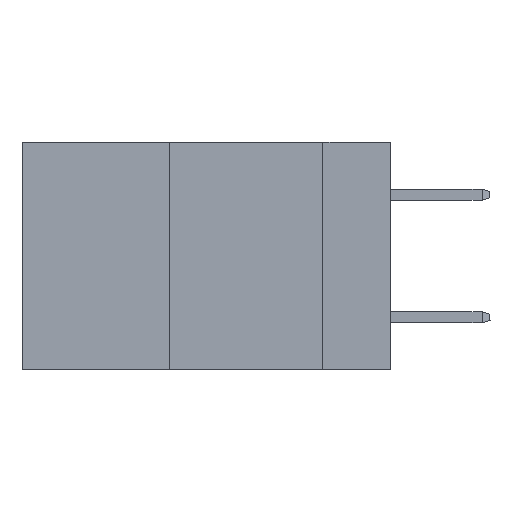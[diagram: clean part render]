
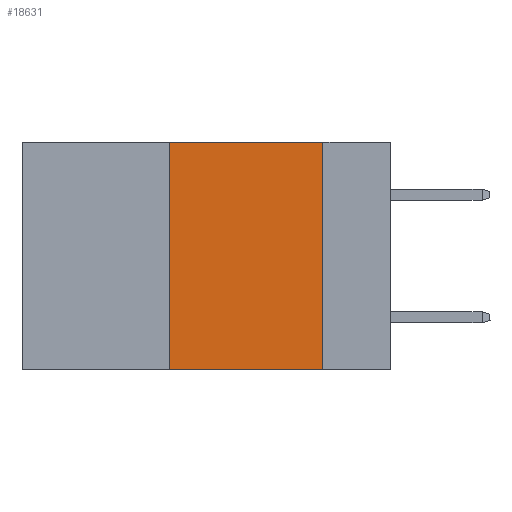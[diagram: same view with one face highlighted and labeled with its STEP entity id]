
A CAD part, left-side view. The second image highlights one B-rep face of the part: STEP entity #18631.
In plain terms, the highlighted planar face has unit normal (-1, 0, 0).
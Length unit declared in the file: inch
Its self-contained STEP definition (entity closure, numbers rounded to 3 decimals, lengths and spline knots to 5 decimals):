
#209 = CARTESIAN_POINT ( 'NONE',  ( 0., 0.6, -0.37 ) ) ;
#716 = EDGE_CURVE ( 'NONE', #15757, #21179, #43046, .T. ) ;
#982 = CARTESIAN_POINT ( 'NONE',  ( 0., 0.11, 0. ) ) ;
#2478 = LINE ( 'NONE', #23327, #38854 ) ;
#2744 = EDGE_LOOP ( 'NONE', ( #33488, #43455, #37711, #19907 ) ) ;
#6216 = CARTESIAN_POINT ( 'NONE',  ( 0., 0.36, -0.37 ) ) ;
#6504 = VERTEX_POINT ( 'NONE', #6216 ) ;
#7935 = VECTOR ( 'NONE', #11816, 39.37008 ) ;
#11541 = CARTESIAN_POINT ( 'NONE',  ( 0., 0.11, -0.37 ) ) ;
#11816 = DIRECTION ( 'NONE',  ( 0., 0., -1. ) ) ;
#14121 = DIRECTION ( 'NONE',  ( 0., -1., 0. ) ) ;
#15757 = VERTEX_POINT ( 'NONE', #33987 ) ;
#18631 = ADVANCED_FACE ( 'NONE', ( #42432 ), #20163, .F. ) ;
#19907 = ORIENTED_EDGE ( 'NONE', *, *, #38723, .T. ) ;
#20163 = PLANE ( 'NONE',  #27413 ) ;
#21179 = VERTEX_POINT ( 'NONE', #11541 ) ;
#22176 = VERTEX_POINT ( 'NONE', #26855 ) ;
#23267 = CARTESIAN_POINT ( 'NONE',  ( 0., 0.36, 0. ) ) ;
#23327 = CARTESIAN_POINT ( 'NONE',  ( 0., 0.6, 0. ) ) ;
#23613 = DIRECTION ( 'NONE',  ( 0., 0., -1. ) ) ;
#25441 = VECTOR ( 'NONE', #36497, 39.37008 ) ;
#26742 = DIRECTION ( 'NONE',  ( 0., -1., 0. ) ) ;
#26855 = CARTESIAN_POINT ( 'NONE',  ( 0., 0.36, 0. ) ) ;
#27211 = VECTOR ( 'NONE', #14121, 39.37008 ) ;
#27413 = AXIS2_PLACEMENT_3D ( 'NONE', #30238, #43678, #23613 ) ;
#30238 = CARTESIAN_POINT ( 'NONE',  ( 0., 0.6, 0. ) ) ;
#32705 = EDGE_CURVE ( 'NONE', #22176, #15757, #2478, .T. ) ;
#33488 = ORIENTED_EDGE ( 'NONE', *, *, #716, .F. ) ;
#33987 = CARTESIAN_POINT ( 'NONE',  ( 0., 0.11, 0. ) ) ;
#35402 = LINE ( 'NONE', #23267, #25441 ) ;
#36497 = DIRECTION ( 'NONE',  ( 0., 0., 1. ) ) ;
#36930 = EDGE_CURVE ( 'NONE', #6504, #22176, #35402, .T. ) ;
#37711 = ORIENTED_EDGE ( 'NONE', *, *, #36930, .F. ) ;
#38723 = EDGE_CURVE ( 'NONE', #6504, #21179, #42883, .T. ) ;
#38854 = VECTOR ( 'NONE', #26742, 39.37008 ) ;
#42432 = FACE_OUTER_BOUND ( 'NONE', #2744, .T. ) ;
#42883 = LINE ( 'NONE', #209, #27211 ) ;
#43046 = LINE ( 'NONE', #982, #7935 ) ;
#43455 = ORIENTED_EDGE ( 'NONE', *, *, #32705, .F. ) ;
#43678 = DIRECTION ( 'NONE',  ( 1., 0., 0. ) ) ;
